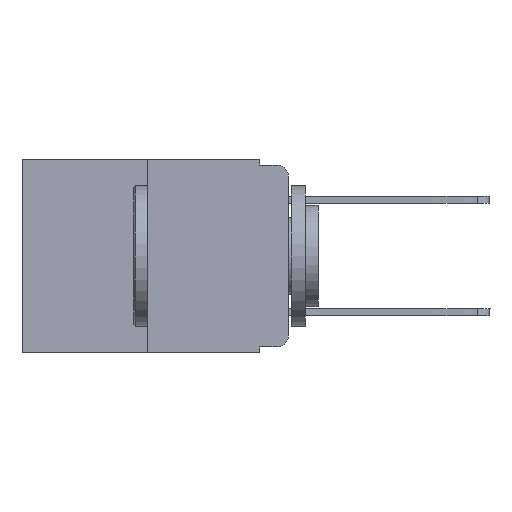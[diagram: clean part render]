
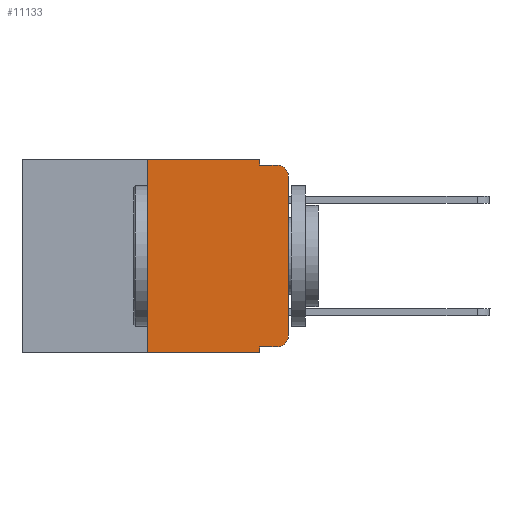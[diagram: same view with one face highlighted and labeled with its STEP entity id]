
A CAD part, left-side view. The second image highlights one B-rep face of the part: STEP entity #11133.
In plain terms, the highlighted planar face has unit normal (-1, 0, 0).
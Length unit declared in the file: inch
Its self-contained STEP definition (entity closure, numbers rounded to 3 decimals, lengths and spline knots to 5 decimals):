
#40 = DIRECTION ( 'NONE',  ( 0., 0., 1. ) ) ;
#65 = VERTEX_POINT ( 'NONE', #8289 ) ;
#226 = CARTESIAN_POINT ( 'NONE',  ( 0., 0.051, -0.343 ) ) ;
#361 = CARTESIAN_POINT ( 'NONE',  ( 0., 0.051, -0.333 ) ) ;
#401 = ORIENTED_EDGE ( 'NONE', *, *, #3381, .F. ) ;
#539 = VERTEX_POINT ( 'NONE', #11216 ) ;
#540 = EDGE_CURVE ( 'NONE', #6083, #6736, #2120, .T. ) ;
#797 = DIRECTION ( 'NONE',  ( 0., 0., -1. ) ) ;
#947 = ORIENTED_EDGE ( 'NONE', *, *, #11369, .F. ) ;
#1155 = CARTESIAN_POINT ( 'NONE',  ( 0., 0.25, 0. ) ) ;
#1294 = AXIS2_PLACEMENT_3D ( 'NONE', #2973, #9268, #7276 ) ;
#1363 = EDGE_CURVE ( 'NONE', #539, #9515, #7916, .T. ) ;
#1619 = EDGE_CURVE ( 'NONE', #9515, #8585, #5061, .T. ) ;
#1853 = LINE ( 'NONE', #9938, #9718 ) ;
#2120 = LINE ( 'NONE', #12283, #3272 ) ;
#2512 = CARTESIAN_POINT ( 'NONE',  ( 0., 0.051, 0. ) ) ;
#2531 = ORIENTED_EDGE ( 'NONE', *, *, #540, .T. ) ;
#2664 = VECTOR ( 'NONE', #10570, 39.37008 ) ;
#2828 = FACE_OUTER_BOUND ( 'NONE', #11534, .T. ) ;
#2973 = CARTESIAN_POINT ( 'NONE',  ( 0., 0.02, -0.313 ) ) ;
#3272 = VECTOR ( 'NONE', #10017, 39.37008 ) ;
#3381 = EDGE_CURVE ( 'NONE', #13035, #65, #7500, .T. ) ;
#3442 = VECTOR ( 'NONE', #9208, 39.37008 ) ;
#3500 = ORIENTED_EDGE ( 'NONE', *, *, #1619, .T. ) ;
#3695 = DIRECTION ( 'NONE',  ( 0., 0., -1. ) ) ;
#3742 = CARTESIAN_POINT ( 'NONE',  ( 0., 0.02, -0.03 ) ) ;
#3777 = CARTESIAN_POINT ( 'NONE',  ( 0., 0.473, -0.343 ) ) ;
#3883 = EDGE_CURVE ( 'NONE', #6083, #5955, #1853, .T. ) ;
#3988 = EDGE_CURVE ( 'NONE', #10641, #5955, #12890, .T. ) ;
#4299 = LINE ( 'NONE', #5169, #3442 ) ;
#4339 = VECTOR ( 'NONE', #12496, 39.37008 ) ;
#4620 = CARTESIAN_POINT ( 'NONE',  ( 0., 0.25, 0. ) ) ;
#4889 = DIRECTION ( 'NONE',  ( 1., 0., 0. ) ) ;
#4959 = AXIS2_PLACEMENT_3D ( 'NONE', #10794, #4889, #3695 ) ;
#5061 = CIRCLE ( 'NONE', #11400, 0.02 ) ;
#5169 = CARTESIAN_POINT ( 'NONE',  ( 0., 0.051, -0.01 ) ) ;
#5516 = LINE ( 'NONE', #2512, #4339 ) ;
#5663 = ORIENTED_EDGE ( 'NONE', *, *, #12255, .F. ) ;
#5933 = CARTESIAN_POINT ( 'NONE',  ( 0., 0., 0. ) ) ;
#5955 = VERTEX_POINT ( 'NONE', #226 ) ;
#6083 = VERTEX_POINT ( 'NONE', #361 ) ;
#6147 = ORIENTED_EDGE ( 'NONE', *, *, #3883, .F. ) ;
#6398 = VERTEX_POINT ( 'NONE', #12369 ) ;
#6514 = CARTESIAN_POINT ( 'NONE',  ( 0., 0.473, 0. ) ) ;
#6532 = DIRECTION ( 'NONE',  ( 0., 0., 1. ) ) ;
#6731 = PLANE ( 'NONE',  #4959 ) ;
#6736 = VERTEX_POINT ( 'NONE', #6954 ) ;
#6936 = EDGE_CURVE ( 'NONE', #6736, #539, #7635, .T. ) ;
#6954 = CARTESIAN_POINT ( 'NONE',  ( 0., 0.02, -0.333 ) ) ;
#7230 = ORIENTED_EDGE ( 'NONE', *, *, #1363, .T. ) ;
#7276 = DIRECTION ( 'NONE',  ( 0., 0., -1. ) ) ;
#7500 = LINE ( 'NONE', #6514, #2664 ) ;
#7584 = LINE ( 'NONE', #4620, #8961 ) ;
#7635 = CIRCLE ( 'NONE', #1294, 0.02 ) ;
#7861 = CARTESIAN_POINT ( 'NONE',  ( 0., 0.02, -0.01 ) ) ;
#7916 = LINE ( 'NONE', #5933, #8414 ) ;
#7931 = ORIENTED_EDGE ( 'NONE', *, *, #6936, .T. ) ;
#8037 = ORIENTED_EDGE ( 'NONE', *, *, #10878, .F. ) ;
#8289 = CARTESIAN_POINT ( 'NONE',  ( 0., 0.051, 0. ) ) ;
#8414 = VECTOR ( 'NONE', #40, 39.37008 ) ;
#8585 = VERTEX_POINT ( 'NONE', #7861 ) ;
#8961 = VECTOR ( 'NONE', #6532, 39.37008 ) ;
#9208 = DIRECTION ( 'NONE',  ( 0., -1., 0. ) ) ;
#9268 = DIRECTION ( 'NONE',  ( -1., 0., 0. ) ) ;
#9515 = VERTEX_POINT ( 'NONE', #11283 ) ;
#9718 = VECTOR ( 'NONE', #797, 39.37008 ) ;
#9938 = CARTESIAN_POINT ( 'NONE',  ( 0., 0.051, 0. ) ) ;
#10017 = DIRECTION ( 'NONE',  ( 0., -1., 0. ) ) ;
#10458 = VECTOR ( 'NONE', #10873, 39.37008 ) ;
#10570 = DIRECTION ( 'NONE',  ( 0., -1., 0. ) ) ;
#10641 = VERTEX_POINT ( 'NONE', #11827 ) ;
#10794 = CARTESIAN_POINT ( 'NONE',  ( 0., 0.473, 0. ) ) ;
#10873 = DIRECTION ( 'NONE',  ( 0., -1., 0. ) ) ;
#10878 = EDGE_CURVE ( 'NONE', #6398, #8585, #4299, .T. ) ;
#11133 = ADVANCED_FACE ( 'NONE', ( #2828 ), #6731, .F. ) ;
#11216 = CARTESIAN_POINT ( 'NONE',  ( 0., 0., -0.313 ) ) ;
#11237 = ORIENTED_EDGE ( 'NONE', *, *, #3988, .T. ) ;
#11283 = CARTESIAN_POINT ( 'NONE',  ( 0., 0., -0.03 ) ) ;
#11369 = EDGE_CURVE ( 'NONE', #10641, #13035, #7584, .T. ) ;
#11400 = AXIS2_PLACEMENT_3D ( 'NONE', #3742, #12713, #11638 ) ;
#11534 = EDGE_LOOP ( 'NONE', ( #7230, #3500, #8037, #5663, #401, #947, #11237, #6147, #2531, #7931 ) ) ;
#11638 = DIRECTION ( 'NONE',  ( 0., 0., -1. ) ) ;
#11827 = CARTESIAN_POINT ( 'NONE',  ( 0., 0.25, -0.343 ) ) ;
#12255 = EDGE_CURVE ( 'NONE', #65, #6398, #5516, .T. ) ;
#12283 = CARTESIAN_POINT ( 'NONE',  ( 0., 0.051, -0.333 ) ) ;
#12369 = CARTESIAN_POINT ( 'NONE',  ( 0., 0.051, -0.01 ) ) ;
#12496 = DIRECTION ( 'NONE',  ( 0., 0., -1. ) ) ;
#12713 = DIRECTION ( 'NONE',  ( -1., 0., 0. ) ) ;
#12890 = LINE ( 'NONE', #3777, #10458 ) ;
#13035 = VERTEX_POINT ( 'NONE', #1155 ) ;
